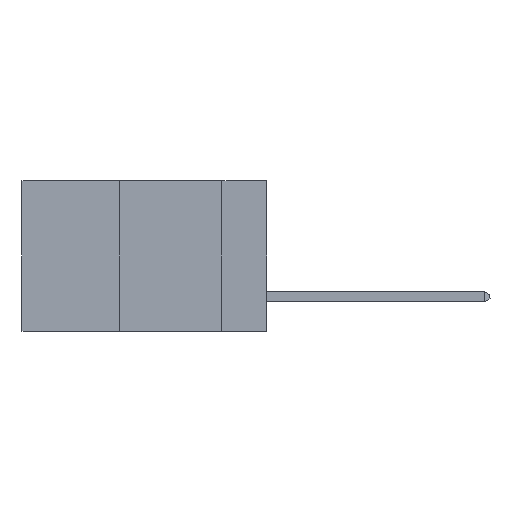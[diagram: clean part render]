
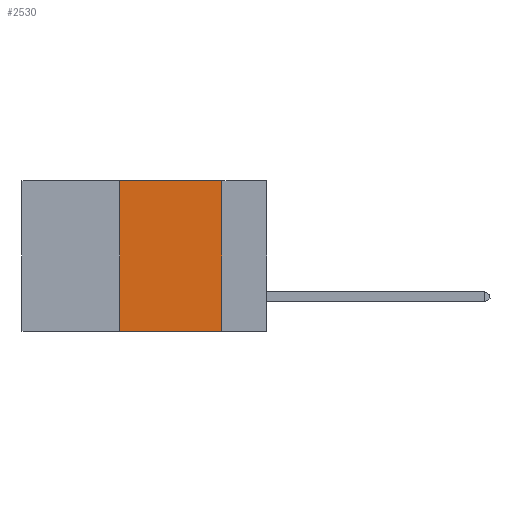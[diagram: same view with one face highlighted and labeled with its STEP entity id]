
A CAD part, left-side view. The second image highlights one B-rep face of the part: STEP entity #2530.
In plain terms, the highlighted planar face has unit normal (-1, 0, 0).
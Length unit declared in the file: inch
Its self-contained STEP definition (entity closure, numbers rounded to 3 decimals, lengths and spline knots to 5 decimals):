
#127 = ORIENTED_EDGE ( 'NONE', *, *, #612, .T. ) ;
#331 = VERTEX_POINT ( 'NONE', #389 ) ;
#389 = CARTESIAN_POINT ( 'NONE',  ( 0., 0.11, -0.37 ) ) ;
#612 = EDGE_CURVE ( 'NONE', #4109, #331, #2672, .T. ) ;
#704 = ORIENTED_EDGE ( 'NONE', *, *, #6789, .F. ) ;
#770 = AXIS2_PLACEMENT_3D ( 'NONE', #3963, #774, #866 ) ;
#774 = DIRECTION ( 'NONE',  ( 1., 0., 0. ) ) ;
#817 = VERTEX_POINT ( 'NONE', #8043 ) ;
#866 = DIRECTION ( 'NONE',  ( 0., 0., -1. ) ) ;
#912 = DIRECTION ( 'NONE',  ( 0., 0., 1. ) ) ;
#1229 = LINE ( 'NONE', #6592, #2501 ) ;
#1276 = LINE ( 'NONE', #2021, #5963 ) ;
#1468 = CARTESIAN_POINT ( 'NONE',  ( 0., 0.11, 0. ) ) ;
#1616 = PLANE ( 'NONE',  #770 ) ;
#2021 = CARTESIAN_POINT ( 'NONE',  ( 0., 0.6, 0. ) ) ;
#2501 = VECTOR ( 'NONE', #912, 39.37008 ) ;
#2530 = ADVANCED_FACE ( 'NONE', ( #2870 ), #1616, .F. ) ;
#2672 = LINE ( 'NONE', #3840, #3680 ) ;
#2870 = FACE_OUTER_BOUND ( 'NONE', #5476, .T. ) ;
#3072 = DIRECTION ( 'NONE',  ( 0., -1., 0. ) ) ;
#3680 = VECTOR ( 'NONE', #3072, 39.37008 ) ;
#3840 = CARTESIAN_POINT ( 'NONE',  ( 0., 0.6, -0.37 ) ) ;
#3861 = DIRECTION ( 'NONE',  ( 0., 0., -1. ) ) ;
#3963 = CARTESIAN_POINT ( 'NONE',  ( 0., 0.6, 0. ) ) ;
#4109 = VERTEX_POINT ( 'NONE', #4308 ) ;
#4308 = CARTESIAN_POINT ( 'NONE',  ( 0., 0.36, -0.37 ) ) ;
#5476 = EDGE_LOOP ( 'NONE', ( #704, #9940, #9582, #127 ) ) ;
#5885 = EDGE_CURVE ( 'NONE', #4109, #817, #1229, .T. ) ;
#5950 = DIRECTION ( 'NONE',  ( 0., -1., 0. ) ) ;
#5963 = VECTOR ( 'NONE', #5950, 39.37008 ) ;
#6592 = CARTESIAN_POINT ( 'NONE',  ( 0., 0.36, 0. ) ) ;
#6784 = VERTEX_POINT ( 'NONE', #1468 ) ;
#6789 = EDGE_CURVE ( 'NONE', #6784, #331, #9697, .T. ) ;
#8043 = CARTESIAN_POINT ( 'NONE',  ( 0., 0.36, 0. ) ) ;
#8348 = VECTOR ( 'NONE', #3861, 39.37008 ) ;
#8537 = CARTESIAN_POINT ( 'NONE',  ( 0., 0.11, 0. ) ) ;
#9582 = ORIENTED_EDGE ( 'NONE', *, *, #5885, .F. ) ;
#9697 = LINE ( 'NONE', #8537, #8348 ) ;
#9837 = EDGE_CURVE ( 'NONE', #817, #6784, #1276, .T. ) ;
#9940 = ORIENTED_EDGE ( 'NONE', *, *, #9837, .F. ) ;
